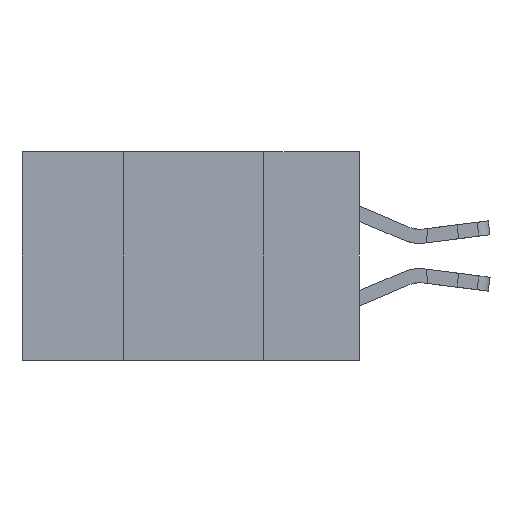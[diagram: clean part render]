
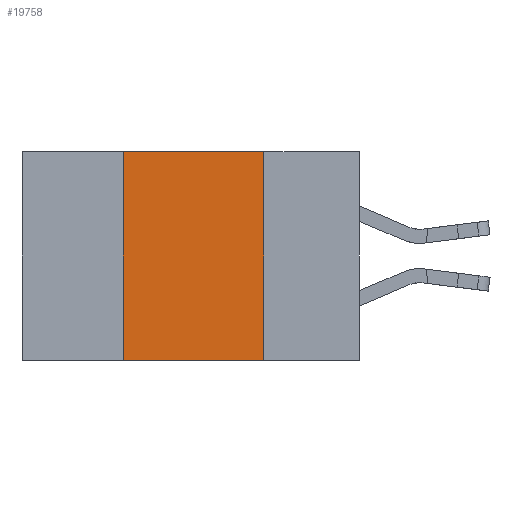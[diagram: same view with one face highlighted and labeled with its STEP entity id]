
A CAD part, left-side view. The second image highlights one B-rep face of the part: STEP entity #19758.
In plain terms, the highlighted planar face has unit normal (-1, 0, 0).
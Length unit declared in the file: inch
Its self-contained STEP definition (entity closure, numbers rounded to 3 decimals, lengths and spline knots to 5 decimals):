
#502 = CARTESIAN_POINT ( 'NONE',  ( 0., 0.17, 0. ) ) ;
#1388 = EDGE_CURVE ( 'NONE', #11517, #14702, #6285, .T. ) ;
#1410 = AXIS2_PLACEMENT_3D ( 'NONE', #11953, #22594, #24446 ) ;
#1485 = VERTEX_POINT ( 'NONE', #20254 ) ;
#1532 = EDGE_LOOP ( 'NONE', ( #23650, #1942, #14509, #9968 ) ) ;
#1690 = VECTOR ( 'NONE', #15345, 39.37008 ) ;
#1942 = ORIENTED_EDGE ( 'NONE', *, *, #1388, .F. ) ;
#2113 = DIRECTION ( 'NONE',  ( 0., 0., 1. ) ) ;
#3459 = VERTEX_POINT ( 'NONE', #16344 ) ;
#3762 = CARTESIAN_POINT ( 'NONE',  ( 0., 0.6, 0. ) ) ;
#5424 = DIRECTION ( 'NONE',  ( 0., 0., -1. ) ) ;
#5889 = CARTESIAN_POINT ( 'NONE',  ( 0., 0.42, 0. ) ) ;
#6285 = LINE ( 'NONE', #3762, #21605 ) ;
#6497 = LINE ( 'NONE', #5889, #8067 ) ;
#6715 = EDGE_CURVE ( 'NONE', #3459, #1485, #19770, .T. ) ;
#7534 = LINE ( 'NONE', #23664, #20934 ) ;
#8067 = VECTOR ( 'NONE', #2113, 39.37008 ) ;
#9968 = ORIENTED_EDGE ( 'NONE', *, *, #6715, .T. ) ;
#11517 = VERTEX_POINT ( 'NONE', #16245 ) ;
#11953 = CARTESIAN_POINT ( 'NONE',  ( 0., 0.6, 0. ) ) ;
#14509 = ORIENTED_EDGE ( 'NONE', *, *, #19036, .F. ) ;
#14702 = VERTEX_POINT ( 'NONE', #502 ) ;
#15345 = DIRECTION ( 'NONE',  ( 0., -1., 0. ) ) ;
#16245 = CARTESIAN_POINT ( 'NONE',  ( 0., 0.42, 0. ) ) ;
#16344 = CARTESIAN_POINT ( 'NONE',  ( 0., 0.42, -0.37 ) ) ;
#17385 = EDGE_CURVE ( 'NONE', #14702, #1485, #7534, .T. ) ;
#17402 = CARTESIAN_POINT ( 'NONE',  ( 0., 0.6, -0.37 ) ) ;
#17738 = DIRECTION ( 'NONE',  ( 0., -1., 0. ) ) ;
#18108 = PLANE ( 'NONE',  #1410 ) ;
#19036 = EDGE_CURVE ( 'NONE', #3459, #11517, #6497, .T. ) ;
#19758 = ADVANCED_FACE ( 'NONE', ( #21737 ), #18108, .F. ) ;
#19770 = LINE ( 'NONE', #17402, #1690 ) ;
#20254 = CARTESIAN_POINT ( 'NONE',  ( 0., 0.17, -0.37 ) ) ;
#20934 = VECTOR ( 'NONE', #5424, 39.37008 ) ;
#21605 = VECTOR ( 'NONE', #17738, 39.37008 ) ;
#21737 = FACE_OUTER_BOUND ( 'NONE', #1532, .T. ) ;
#22594 = DIRECTION ( 'NONE',  ( 1., 0., 0. ) ) ;
#23650 = ORIENTED_EDGE ( 'NONE', *, *, #17385, .F. ) ;
#23664 = CARTESIAN_POINT ( 'NONE',  ( 0., 0.17, 0. ) ) ;
#24446 = DIRECTION ( 'NONE',  ( 0., 0., -1. ) ) ;
